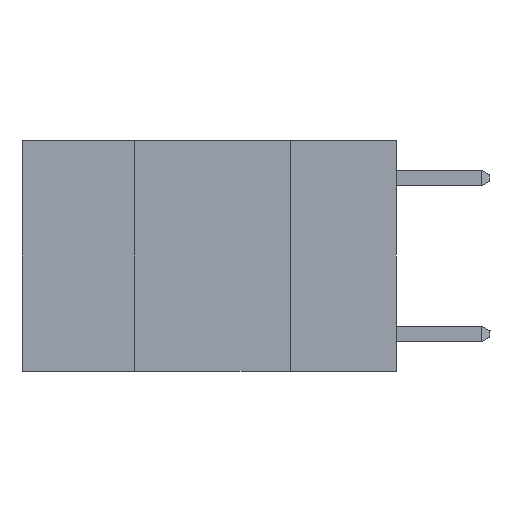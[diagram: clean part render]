
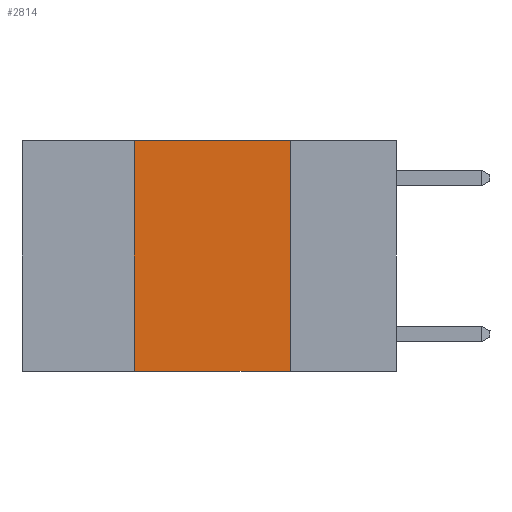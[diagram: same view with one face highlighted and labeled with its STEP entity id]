
A CAD part, left-side view. The second image highlights one B-rep face of the part: STEP entity #2814.
In plain terms, the highlighted planar face has unit normal (-1, 0, 0).
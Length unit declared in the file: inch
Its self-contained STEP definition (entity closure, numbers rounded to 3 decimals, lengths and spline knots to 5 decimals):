
#264 = CARTESIAN_POINT ( 'NONE',  ( 0., 0.6, 0. ) ) ;
#2814 = ADVANCED_FACE ( 'NONE', ( #10514 ), #25499, .F. ) ;
#4328 = LINE ( 'NONE', #24032, #4634 ) ;
#4634 = VECTOR ( 'NONE', #23865, 39.37008 ) ;
#4808 = EDGE_CURVE ( 'NONE', #29179, #17683, #6237, .T. ) ;
#5091 = VERTEX_POINT ( 'NONE', #15018 ) ;
#5141 = LINE ( 'NONE', #5302, #28000 ) ;
#5302 = CARTESIAN_POINT ( 'NONE',  ( 0., 0.42, 0. ) ) ;
#6237 = LINE ( 'NONE', #25947, #10946 ) ;
#10514 = FACE_OUTER_BOUND ( 'NONE', #30678, .T. ) ;
#10703 = ORIENTED_EDGE ( 'NONE', *, *, #4808, .T. ) ;
#10737 = DIRECTION ( 'NONE',  ( 0., 0., -1. ) ) ;
#10946 = VECTOR ( 'NONE', #16178, 39.37008 ) ;
#11626 = ORIENTED_EDGE ( 'NONE', *, *, #22621, .F. ) ;
#13065 = CARTESIAN_POINT ( 'NONE',  ( 0., 0.17, -0.37 ) ) ;
#15018 = CARTESIAN_POINT ( 'NONE',  ( 0., 0.17, 0. ) ) ;
#15413 = DIRECTION ( 'NONE',  ( 0., 0., -1. ) ) ;
#15490 = VECTOR ( 'NONE', #10737, 39.37008 ) ;
#16178 = DIRECTION ( 'NONE',  ( 0., -1., 0. ) ) ;
#16810 = VERTEX_POINT ( 'NONE', #28473 ) ;
#17683 = VERTEX_POINT ( 'NONE', #13065 ) ;
#17902 = CARTESIAN_POINT ( 'NONE',  ( 0., 0.17, 0. ) ) ;
#21831 = CARTESIAN_POINT ( 'NONE',  ( 0., 0.42, -0.37 ) ) ;
#22365 = EDGE_CURVE ( 'NONE', #5091, #17683, #30941, .T. ) ;
#22621 = EDGE_CURVE ( 'NONE', #29179, #16810, #5141, .T. ) ;
#22731 = DIRECTION ( 'NONE',  ( 1., 0., 0. ) ) ;
#23865 = DIRECTION ( 'NONE',  ( 0., -1., 0. ) ) ;
#24032 = CARTESIAN_POINT ( 'NONE',  ( 0., 0.6, 0. ) ) ;
#24135 = EDGE_CURVE ( 'NONE', #16810, #5091, #4328, .T. ) ;
#25499 = PLANE ( 'NONE',  #25503 ) ;
#25503 = AXIS2_PLACEMENT_3D ( 'NONE', #264, #22731, #15413 ) ;
#25947 = CARTESIAN_POINT ( 'NONE',  ( 0., 0.6, -0.37 ) ) ;
#26445 = ORIENTED_EDGE ( 'NONE', *, *, #22365, .F. ) ;
#26962 = ORIENTED_EDGE ( 'NONE', *, *, #24135, .F. ) ;
#27786 = DIRECTION ( 'NONE',  ( 0., 0., 1. ) ) ;
#28000 = VECTOR ( 'NONE', #27786, 39.37008 ) ;
#28473 = CARTESIAN_POINT ( 'NONE',  ( 0., 0.42, 0. ) ) ;
#29179 = VERTEX_POINT ( 'NONE', #21831 ) ;
#30678 = EDGE_LOOP ( 'NONE', ( #26445, #26962, #11626, #10703 ) ) ;
#30941 = LINE ( 'NONE', #17902, #15490 ) ;
